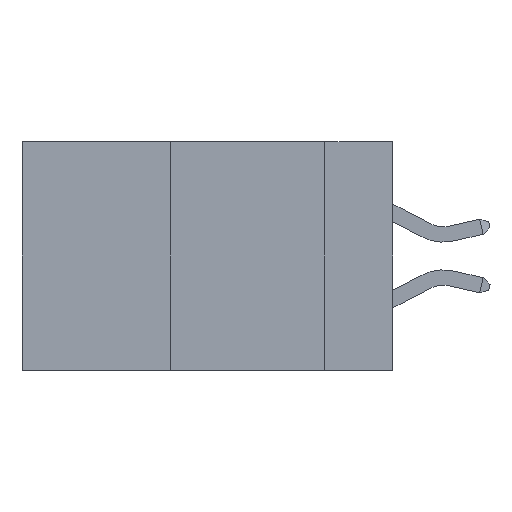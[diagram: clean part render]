
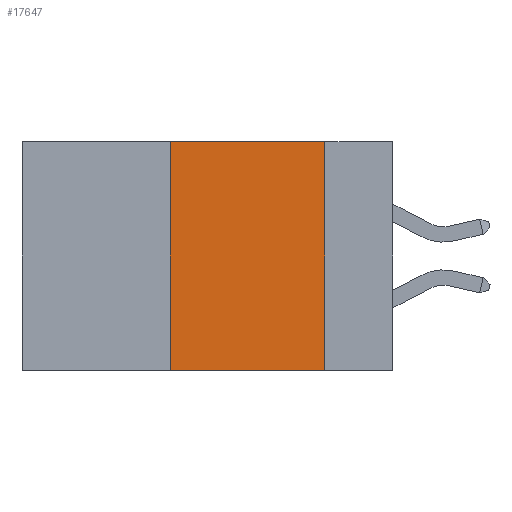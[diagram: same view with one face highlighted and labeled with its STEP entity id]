
A CAD part, left-side view. The second image highlights one B-rep face of the part: STEP entity #17647.
In plain terms, the highlighted planar face has unit normal (-1, 0, 0).
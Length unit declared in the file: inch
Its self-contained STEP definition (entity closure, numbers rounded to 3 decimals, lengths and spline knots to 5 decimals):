
#558 = EDGE_CURVE ( 'NONE', #8236, #6022, #6527, .T. ) ;
#2832 = EDGE_LOOP ( 'NONE', ( #17895, #15447, #13241, #23648 ) ) ;
#3494 = DIRECTION ( 'NONE',  ( 0., 0., -1. ) ) ;
#3967 = EDGE_CURVE ( 'NONE', #8236, #19160, #19039, .T. ) ;
#4362 = LINE ( 'NONE', #9113, #9049 ) ;
#4953 = VECTOR ( 'NONE', #7535, 39.37008 ) ;
#5671 = CARTESIAN_POINT ( 'NONE',  ( 0., 0.6, -0.37 ) ) ;
#5999 = CARTESIAN_POINT ( 'NONE',  ( 0., 0.11, -0.37 ) ) ;
#6022 = VERTEX_POINT ( 'NONE', #5999 ) ;
#6063 = DIRECTION ( 'NONE',  ( 0., 0., 1. ) ) ;
#6527 = LINE ( 'NONE', #5671, #4953 ) ;
#7447 = AXIS2_PLACEMENT_3D ( 'NONE', #13550, #15555, #3494 ) ;
#7528 = CARTESIAN_POINT ( 'NONE',  ( 0., 0.36, 0. ) ) ;
#7535 = DIRECTION ( 'NONE',  ( 0., -1., 0. ) ) ;
#8236 = VERTEX_POINT ( 'NONE', #13761 ) ;
#9049 = VECTOR ( 'NONE', #23173, 39.37008 ) ;
#9113 = CARTESIAN_POINT ( 'NONE',  ( 0., 0.6, 0. ) ) ;
#10240 = CARTESIAN_POINT ( 'NONE',  ( 0., 0.36, 0. ) ) ;
#10856 = VERTEX_POINT ( 'NONE', #11625 ) ;
#11625 = CARTESIAN_POINT ( 'NONE',  ( 0., 0.11, 0. ) ) ;
#13241 = ORIENTED_EDGE ( 'NONE', *, *, #3967, .F. ) ;
#13550 = CARTESIAN_POINT ( 'NONE',  ( 0., 0.6, 0. ) ) ;
#13761 = CARTESIAN_POINT ( 'NONE',  ( 0., 0.36, -0.37 ) ) ;
#13990 = VECTOR ( 'NONE', #6063, 39.37008 ) ;
#15447 = ORIENTED_EDGE ( 'NONE', *, *, #17306, .F. ) ;
#15555 = DIRECTION ( 'NONE',  ( 1., 0., 0. ) ) ;
#16231 = DIRECTION ( 'NONE',  ( 0., 0., -1. ) ) ;
#16406 = CARTESIAN_POINT ( 'NONE',  ( 0., 0.11, 0. ) ) ;
#16964 = EDGE_CURVE ( 'NONE', #10856, #6022, #24816, .T. ) ;
#17306 = EDGE_CURVE ( 'NONE', #19160, #10856, #4362, .T. ) ;
#17647 = ADVANCED_FACE ( 'NONE', ( #19097 ), #25586, .F. ) ;
#17895 = ORIENTED_EDGE ( 'NONE', *, *, #16964, .F. ) ;
#19039 = LINE ( 'NONE', #7528, #13990 ) ;
#19097 = FACE_OUTER_BOUND ( 'NONE', #2832, .T. ) ;
#19160 = VERTEX_POINT ( 'NONE', #10240 ) ;
#23173 = DIRECTION ( 'NONE',  ( 0., -1., 0. ) ) ;
#23648 = ORIENTED_EDGE ( 'NONE', *, *, #558, .T. ) ;
#24167 = VECTOR ( 'NONE', #16231, 39.37008 ) ;
#24816 = LINE ( 'NONE', #16406, #24167 ) ;
#25586 = PLANE ( 'NONE',  #7447 ) ;
